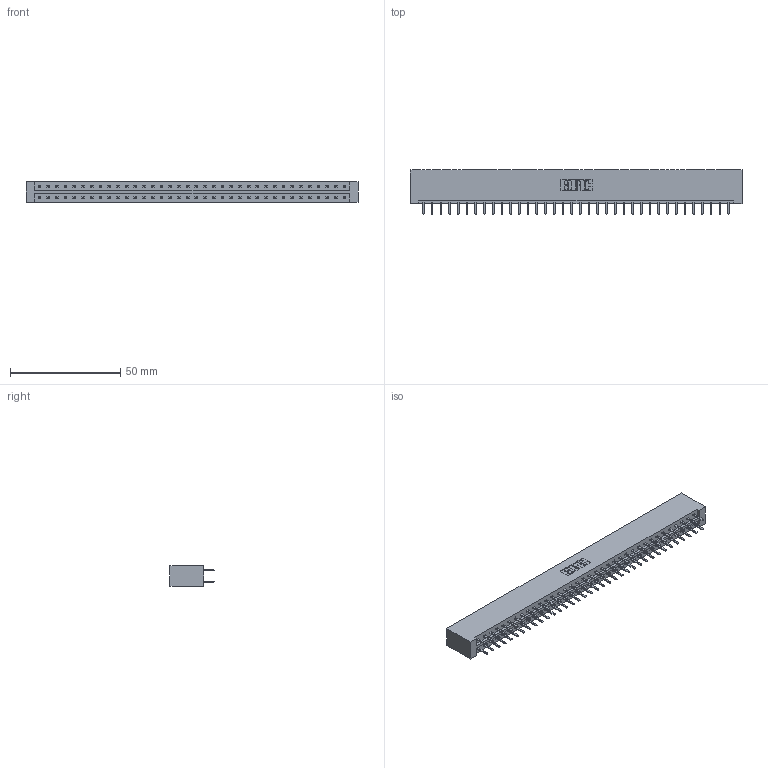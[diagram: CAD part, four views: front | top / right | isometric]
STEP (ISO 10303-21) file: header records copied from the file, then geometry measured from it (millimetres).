
FILE_DESCRIPTION (( 'STEP AP203' ), '1' );
FILE_NAME ('833-072-520-201.STEP', '2020-06-05T13:37:26', ( '' ), ( '' ), 'SwSTEP 2.0', 'SolidWorks 2020', '' );
FILE_SCHEMA (( 'CONFIG_CONTROL_DESIGN' ));
Length unit declared in the file: inch
Products named in the file (3): 345-292-001_345-293-120; 833 Part_Lugless; 833-072-520-201
Assembly tree (73 placements, depth 2):
  833-072-520-201
    833 Part_Lugless
    345-292-001_345-293-120  x72
Bounding box: 150.9 x 20.02 x 9.4 mm (x, y, z)
Volume: 15950.6 mm3; surface area: 18733.7 mm2
Topology: 73 solids, 73 shells, 4138 faces, 12023 edges, 7822 vertices
Faces by surface type: plane 2802, cylinder 1336
Entity records: 23773 total; most frequent: CARTESIAN_POINT 3958, ORIENTED_EDGE 3882, DIRECTION 3373, EDGE_CURVE 1941, VECTOR 1817, LINE 1817, VERTEX_POINT 1290, AXIS2_PLACEMENT_3D 778
